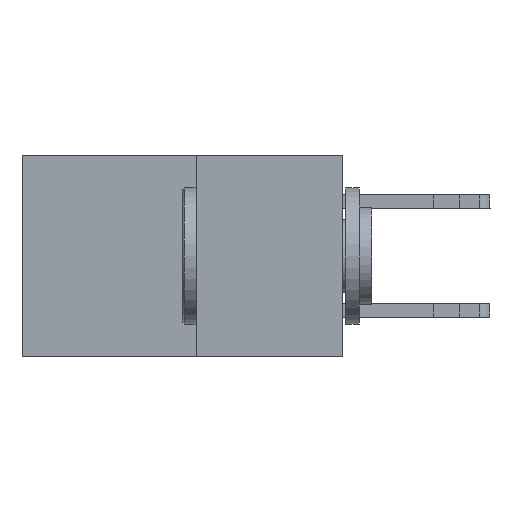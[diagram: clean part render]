
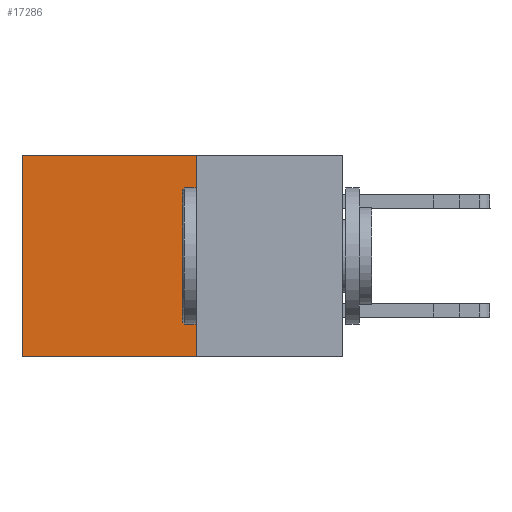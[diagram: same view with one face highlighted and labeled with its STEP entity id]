
A CAD part, left-side view. The second image highlights one B-rep face of the part: STEP entity #17286.
In plain terms, the highlighted planar face has unit normal (-1, 0, 0).
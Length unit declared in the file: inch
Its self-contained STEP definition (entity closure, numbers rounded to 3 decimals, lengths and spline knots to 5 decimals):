
#791 = VERTEX_POINT ( 'NONE', #18390 ) ;
#3170 = DIRECTION ( 'NONE',  ( 0., 1., 0. ) ) ;
#3710 = VECTOR ( 'NONE', #10835, 39.37008 ) ;
#4351 = CARTESIAN_POINT ( 'NONE',  ( 0.277, 0.59, 0. ) ) ;
#4699 = EDGE_CURVE ( 'NONE', #13678, #791, #18552, .T. ) ;
#5167 = VERTEX_POINT ( 'NONE', #16111 ) ;
#5236 = EDGE_CURVE ( 'NONE', #791, #5167, #17700, .T. ) ;
#5520 = AXIS2_PLACEMENT_3D ( 'NONE', #13255, #16149, #7507 ) ;
#6018 = EDGE_LOOP ( 'NONE', ( #6623, #7543, #7921, #9026 ) ) ;
#6254 = VECTOR ( 'NONE', #16531, 39.37008 ) ;
#6311 = VECTOR ( 'NONE', #3170, 39.37008 ) ;
#6623 = ORIENTED_EDGE ( 'NONE', *, *, #16184, .T. ) ;
#7394 = PLANE ( 'NONE',  #5520 ) ;
#7507 = DIRECTION ( 'NONE',  ( 0., 0., -1. ) ) ;
#7543 = ORIENTED_EDGE ( 'NONE', *, *, #5236, .F. ) ;
#7794 = FACE_OUTER_BOUND ( 'NONE', #6018, .T. ) ;
#7921 = ORIENTED_EDGE ( 'NONE', *, *, #4699, .F. ) ;
#9026 = ORIENTED_EDGE ( 'NONE', *, *, #13790, .T. ) ;
#10835 = DIRECTION ( 'NONE',  ( 0., 0., -1. ) ) ;
#11004 = CARTESIAN_POINT ( 'NONE',  ( 0.277, 0.27, -0.37 ) ) ;
#11180 = DIRECTION ( 'NONE',  ( 0., 0., -1. ) ) ;
#11443 = CARTESIAN_POINT ( 'NONE',  ( 0.277, 0.27, 0. ) ) ;
#11632 = LINE ( 'NONE', #15443, #15000 ) ;
#11682 = VERTEX_POINT ( 'NONE', #4351 ) ;
#13255 = CARTESIAN_POINT ( 'NONE',  ( 0.277, 0.27, -0.37 ) ) ;
#13505 = LINE ( 'NONE', #14830, #6311 ) ;
#13678 = VERTEX_POINT ( 'NONE', #11443 ) ;
#13790 = EDGE_CURVE ( 'NONE', #13678, #11682, #13505, .T. ) ;
#14830 = CARTESIAN_POINT ( 'NONE',  ( 0.277, 0.27, 0. ) ) ;
#14895 = CARTESIAN_POINT ( 'NONE',  ( 0.277, 0.27, -0.37 ) ) ;
#15000 = VECTOR ( 'NONE', #11180, 39.37008 ) ;
#15443 = CARTESIAN_POINT ( 'NONE',  ( 0.277, 0.59, -0.37 ) ) ;
#16111 = CARTESIAN_POINT ( 'NONE',  ( 0.277, 0.59, -0.37 ) ) ;
#16149 = DIRECTION ( 'NONE',  ( 1., 0., 0. ) ) ;
#16184 = EDGE_CURVE ( 'NONE', #11682, #5167, #11632, .T. ) ;
#16531 = DIRECTION ( 'NONE',  ( 0., 1., 0. ) ) ;
#17286 = ADVANCED_FACE ( 'NONE', ( #7794 ), #7394, .F. ) ;
#17700 = LINE ( 'NONE', #14895, #6254 ) ;
#18390 = CARTESIAN_POINT ( 'NONE',  ( 0.277, 0.27, -0.37 ) ) ;
#18552 = LINE ( 'NONE', #11004, #3710 ) ;
